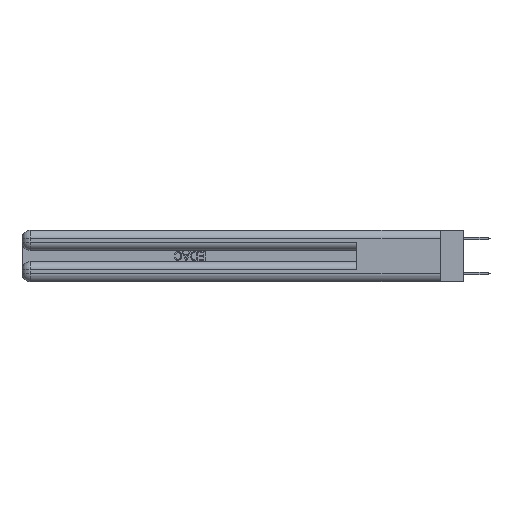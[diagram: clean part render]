
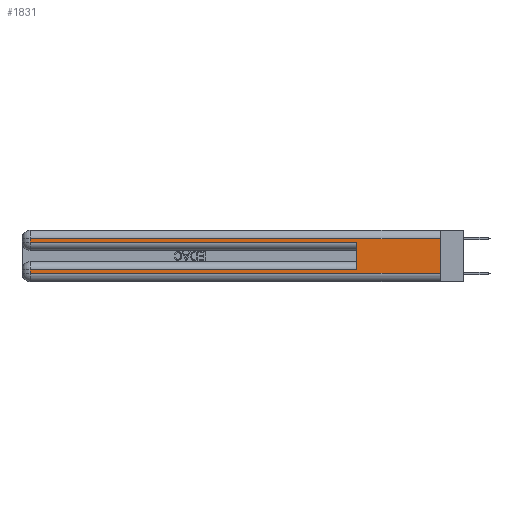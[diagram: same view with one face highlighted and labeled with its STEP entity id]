
A CAD part, left-side view. The second image highlights one B-rep face of the part: STEP entity #1831.
In plain terms, the highlighted planar face has unit normal (-1, 0, 0).
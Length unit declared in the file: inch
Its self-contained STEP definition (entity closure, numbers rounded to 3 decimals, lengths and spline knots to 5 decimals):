
#136 = VERTEX_POINT ( 'NONE', #23591 ) ;
#851 = CARTESIAN_POINT ( 'NONE',  ( 0., 0., 0.285 ) ) ;
#974 = CARTESIAN_POINT ( 'NONE',  ( 0., 0., 0.37 ) ) ;
#1299 = VERTEX_POINT ( 'NONE', #16249 ) ;
#1425 = VERTEX_POINT ( 'NONE', #10362 ) ;
#1831 = ADVANCED_FACE ( 'NONE', ( #13401 ), #24759, .F. ) ;
#2944 = VERTEX_POINT ( 'NONE', #21876 ) ;
#4142 = ORIENTED_EDGE ( 'NONE', *, *, #5346, .F. ) ;
#4219 = EDGE_CURVE ( 'NONE', #1425, #1299, #14066, .T. ) ;
#4236 = VECTOR ( 'NONE', #14891, 39.37008 ) ;
#4411 = EDGE_CURVE ( 'NONE', #11390, #136, #18140, .T. ) ;
#4579 = VECTOR ( 'NONE', #18547, 39.37008 ) ;
#4728 = DIRECTION ( 'NONE',  ( 0., 0., -1. ) ) ;
#4743 = CARTESIAN_POINT ( 'NONE',  ( 0., 0., 0.31 ) ) ;
#5230 = DIRECTION ( 'NONE',  ( 0., -1., 0. ) ) ;
#5346 = EDGE_CURVE ( 'NONE', #11415, #2944, #9052, .T. ) ;
#6338 = VECTOR ( 'NONE', #5230, 39.37008 ) ;
#6374 = EDGE_CURVE ( 'NONE', #136, #2944, #21330, .T. ) ;
#6424 = VECTOR ( 'NONE', #6828, 39.37008 ) ;
#6828 = DIRECTION ( 'NONE',  ( 0., 0., 1. ) ) ;
#6932 = DIRECTION ( 'NONE',  ( 1., 0., 0. ) ) ;
#7066 = VECTOR ( 'NONE', #27952, 39.37008 ) ;
#8114 = CARTESIAN_POINT ( 'NONE',  ( 0., 0., 0.31 ) ) ;
#8204 = VECTOR ( 'NONE', #12241, 39.37008 ) ;
#9052 = LINE ( 'NONE', #11405, #6424 ) ;
#9247 = LINE ( 'NONE', #24857, #28931 ) ;
#10344 = CARTESIAN_POINT ( 'NONE',  ( 0., 2.94, 0.37 ) ) ;
#10362 = CARTESIAN_POINT ( 'NONE',  ( 0., 2.94, 0.06 ) ) ;
#11080 = CARTESIAN_POINT ( 'NONE',  ( 0., 2.94, 0.37 ) ) ;
#11390 = VERTEX_POINT ( 'NONE', #25976 ) ;
#11405 = CARTESIAN_POINT ( 'NONE',  ( 0., 0.6, 0.145 ) ) ;
#11415 = VERTEX_POINT ( 'NONE', #12276 ) ;
#12241 = DIRECTION ( 'NONE',  ( 0., 0., -1. ) ) ;
#12276 = CARTESIAN_POINT ( 'NONE',  ( 0., 0.6, 0.085 ) ) ;
#12539 = LINE ( 'NONE', #8114, #4236 ) ;
#12992 = VERTEX_POINT ( 'NONE', #15464 ) ;
#13401 = FACE_OUTER_BOUND ( 'NONE', #14642, .T. ) ;
#13936 = DIRECTION ( 'NONE',  ( 0., 1., 0. ) ) ;
#14027 = EDGE_CURVE ( 'NONE', #12992, #1425, #21526, .T. ) ;
#14033 = ORIENTED_EDGE ( 'NONE', *, *, #22555, .F. ) ;
#14066 = LINE ( 'NONE', #23041, #6338 ) ;
#14642 = EDGE_LOOP ( 'NONE', ( #14033, #16514, #14751, #16051, #4142, #24973, #16180, #28930 ) ) ;
#14751 = ORIENTED_EDGE ( 'NONE', *, *, #4411, .T. ) ;
#14891 = DIRECTION ( 'NONE',  ( 0., 1., 0. ) ) ;
#15464 = CARTESIAN_POINT ( 'NONE',  ( 0., 2.94, 0.085 ) ) ;
#16051 = ORIENTED_EDGE ( 'NONE', *, *, #6374, .T. ) ;
#16180 = ORIENTED_EDGE ( 'NONE', *, *, #14027, .T. ) ;
#16249 = CARTESIAN_POINT ( 'NONE',  ( 0., 0., 0.06 ) ) ;
#16514 = ORIENTED_EDGE ( 'NONE', *, *, #20426, .T. ) ;
#17014 = VERTEX_POINT ( 'NONE', #4743 ) ;
#18140 = LINE ( 'NONE', #11080, #23256 ) ;
#18547 = DIRECTION ( 'NONE',  ( 0., -1., 0. ) ) ;
#20426 = EDGE_CURVE ( 'NONE', #17014, #11390, #12539, .T. ) ;
#21330 = LINE ( 'NONE', #851, #4579 ) ;
#21526 = LINE ( 'NONE', #10344, #8204 ) ;
#21876 = CARTESIAN_POINT ( 'NONE',  ( 0., 0.6, 0.285 ) ) ;
#22407 = DIRECTION ( 'NONE',  ( 0., 0., -1. ) ) ;
#22555 = EDGE_CURVE ( 'NONE', #17014, #1299, #25887, .T. ) ;
#22842 = AXIS2_PLACEMENT_3D ( 'NONE', #27279, #6932, #22407 ) ;
#23041 = CARTESIAN_POINT ( 'NONE',  ( 0., 0., 0.06 ) ) ;
#23256 = VECTOR ( 'NONE', #4728, 39.37008 ) ;
#23591 = CARTESIAN_POINT ( 'NONE',  ( 0., 2.94, 0.285 ) ) ;
#24759 = PLANE ( 'NONE',  #22842 ) ;
#24857 = CARTESIAN_POINT ( 'NONE',  ( 0., 0., 0.085 ) ) ;
#24973 = ORIENTED_EDGE ( 'NONE', *, *, #27752, .T. ) ;
#25887 = LINE ( 'NONE', #974, #7066 ) ;
#25976 = CARTESIAN_POINT ( 'NONE',  ( 0., 2.94, 0.31 ) ) ;
#27279 = CARTESIAN_POINT ( 'NONE',  ( 0., 0., 0.37 ) ) ;
#27752 = EDGE_CURVE ( 'NONE', #11415, #12992, #9247, .T. ) ;
#27952 = DIRECTION ( 'NONE',  ( 0., 0., -1. ) ) ;
#28930 = ORIENTED_EDGE ( 'NONE', *, *, #4219, .T. ) ;
#28931 = VECTOR ( 'NONE', #13936, 39.37008 ) ;
